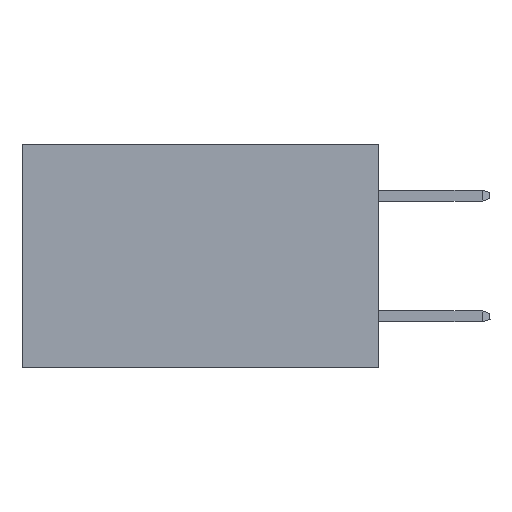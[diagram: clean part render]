
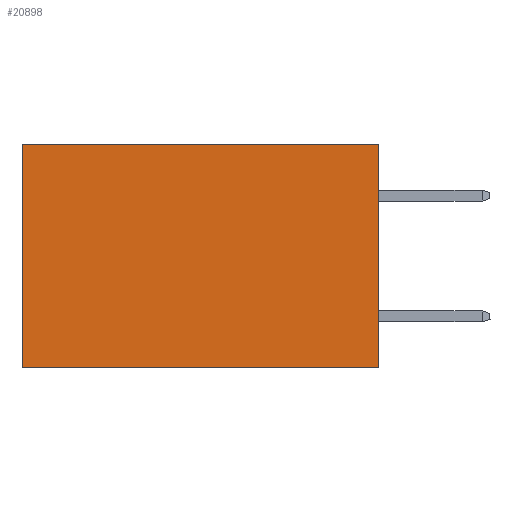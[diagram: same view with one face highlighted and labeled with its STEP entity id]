
A CAD part, left-side view. The second image highlights one B-rep face of the part: STEP entity #20898.
In plain terms, the highlighted planar face has unit normal (-1, 0, 0).
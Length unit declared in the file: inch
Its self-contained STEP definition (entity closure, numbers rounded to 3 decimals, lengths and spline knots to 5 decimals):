
#253 = CARTESIAN_POINT ( 'NONE',  ( 0.277, 0., -0.37 ) ) ;
#1930 = ORIENTED_EDGE ( 'NONE', *, *, #10997, .T. ) ;
#2984 = VERTEX_POINT ( 'NONE', #17522 ) ;
#3451 = DIRECTION ( 'NONE',  ( 0., 0., -1. ) ) ;
#3926 = DIRECTION ( 'NONE',  ( 0., 1., 0. ) ) ;
#4372 = CARTESIAN_POINT ( 'NONE',  ( 0.277, 0., -0.37 ) ) ;
#5431 = CARTESIAN_POINT ( 'NONE',  ( 0.277, 0., 0. ) ) ;
#7076 = VECTOR ( 'NONE', #14231, 39.37008 ) ;
#8008 = VECTOR ( 'NONE', #11644, 39.37008 ) ;
#8215 = LINE ( 'NONE', #253, #16958 ) ;
#8608 = EDGE_CURVE ( 'NONE', #2984, #16867, #17289, .T. ) ;
#8979 = VERTEX_POINT ( 'NONE', #10638 ) ;
#10312 = ORIENTED_EDGE ( 'NONE', *, *, #8608, .F. ) ;
#10483 = EDGE_CURVE ( 'NONE', #16867, #8979, #8215, .T. ) ;
#10638 = CARTESIAN_POINT ( 'NONE',  ( 0.277, 0.59, -0.37 ) ) ;
#10684 = EDGE_CURVE ( 'NONE', #15071, #8979, #13127, .T. ) ;
#10997 = EDGE_CURVE ( 'NONE', #2984, #15071, #20350, .T. ) ;
#11411 = ORIENTED_EDGE ( 'NONE', *, *, #10684, .T. ) ;
#11644 = DIRECTION ( 'NONE',  ( 0., 0., -1. ) ) ;
#12252 = PLANE ( 'NONE',  #14092 ) ;
#13127 = LINE ( 'NONE', #16983, #22206 ) ;
#13798 = CARTESIAN_POINT ( 'NONE',  ( 0.277, 0., -0.37 ) ) ;
#14002 = DIRECTION ( 'NONE',  ( 1., 0., 0. ) ) ;
#14092 = AXIS2_PLACEMENT_3D ( 'NONE', #20733, #14002, #3451 ) ;
#14231 = DIRECTION ( 'NONE',  ( 0., 1., 0. ) ) ;
#15071 = VERTEX_POINT ( 'NONE', #20519 ) ;
#15822 = FACE_OUTER_BOUND ( 'NONE', #16003, .T. ) ;
#16003 = EDGE_LOOP ( 'NONE', ( #11411, #17973, #10312, #1930 ) ) ;
#16867 = VERTEX_POINT ( 'NONE', #4372 ) ;
#16958 = VECTOR ( 'NONE', #3926, 39.37008 ) ;
#16983 = CARTESIAN_POINT ( 'NONE',  ( 0.277, 0.59, -0.37 ) ) ;
#17289 = LINE ( 'NONE', #13798, #8008 ) ;
#17522 = CARTESIAN_POINT ( 'NONE',  ( 0.277, 0., 0. ) ) ;
#17973 = ORIENTED_EDGE ( 'NONE', *, *, #10483, .F. ) ;
#20006 = DIRECTION ( 'NONE',  ( 0., 0., -1. ) ) ;
#20350 = LINE ( 'NONE', #5431, #7076 ) ;
#20519 = CARTESIAN_POINT ( 'NONE',  ( 0.277, 0.59, 0. ) ) ;
#20733 = CARTESIAN_POINT ( 'NONE',  ( 0.277, 0., -0.37 ) ) ;
#20898 = ADVANCED_FACE ( 'NONE', ( #15822 ), #12252, .F. ) ;
#22206 = VECTOR ( 'NONE', #20006, 39.37008 ) ;
